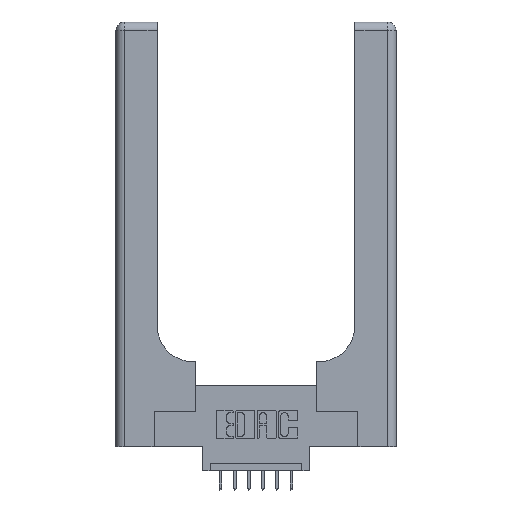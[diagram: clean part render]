
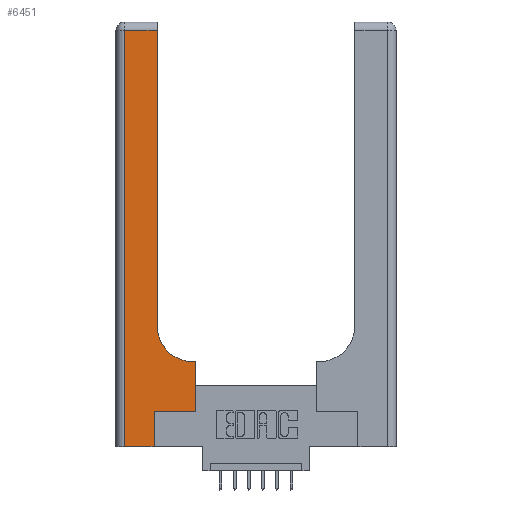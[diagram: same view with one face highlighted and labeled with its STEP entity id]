
A CAD part, top view. The second image highlights one B-rep face of the part: STEP entity #6451.
In plain terms, the highlighted planar face has unit normal (0, 0, 1).
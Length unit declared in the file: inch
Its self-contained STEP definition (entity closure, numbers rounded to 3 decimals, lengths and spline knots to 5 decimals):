
#187 = VECTOR ( 'NONE', #1304, 39.37008 ) ;
#385 = DIRECTION ( 'NONE',  ( -1., 0., 0. ) ) ;
#401 = LINE ( 'NONE', #9521, #187 ) ;
#418 = VECTOR ( 'NONE', #4972, 39.37008 ) ;
#908 = ORIENTED_EDGE ( 'NONE', *, *, #1554, .T. ) ;
#963 = VECTOR ( 'NONE', #2207, 39.37008 ) ;
#1245 = VECTOR ( 'NONE', #10351, 39.37008 ) ;
#1304 = DIRECTION ( 'NONE',  ( -1., 0., 0. ) ) ;
#1554 = EDGE_CURVE ( 'NONE', #9385, #5595, #4899, .T. ) ;
#1590 = VECTOR ( 'NONE', #8329, 39.37008 ) ;
#1761 = EDGE_LOOP ( 'NONE', ( #10314, #908, #6744, #7640, #12966, #4471, #8018, #3297, #11450 ) ) ;
#2207 = DIRECTION ( 'NONE',  ( 0., -1., 0. ) ) ;
#2430 = VECTOR ( 'NONE', #12287, 39.37008 ) ;
#2512 = CARTESIAN_POINT ( 'NONE',  ( 0.5415, 0.6, 0.37 ) ) ;
#2576 = CARTESIAN_POINT ( 'NONE',  ( 0.5585, 0.25, 0.37 ) ) ;
#2887 = CARTESIAN_POINT ( 'NONE',  ( 0.269, 0., 0.37 ) ) ;
#2919 = VERTEX_POINT ( 'NONE', #9083 ) ;
#3297 = ORIENTED_EDGE ( 'NONE', *, *, #8586, .T. ) ;
#3600 = CARTESIAN_POINT ( 'NONE',  ( 0.5585, 0.25, 0.37 ) ) ;
#4205 = VERTEX_POINT ( 'NONE', #2512 ) ;
#4418 = EDGE_CURVE ( 'NONE', #7313, #6484, #11014, .T. ) ;
#4419 = EDGE_CURVE ( 'NONE', #5595, #7313, #14674, .T. ) ;
#4471 = ORIENTED_EDGE ( 'NONE', *, *, #13167, .T. ) ;
#4771 = EDGE_CURVE ( 'NONE', #4205, #10143, #4777, .T. ) ;
#4777 = CIRCLE ( 'NONE', #7892, 0.25 ) ;
#4882 = CARTESIAN_POINT ( 'NONE',  ( 0.06, 0., 0.37 ) ) ;
#4899 = LINE ( 'NONE', #6180, #418 ) ;
#4972 = DIRECTION ( 'NONE',  ( -1., 0., 0. ) ) ;
#5291 = CARTESIAN_POINT ( 'NONE',  ( 0.06, 2.94, 0.37 ) ) ;
#5488 = LINE ( 'NONE', #8023, #9091 ) ;
#5595 = VERTEX_POINT ( 'NONE', #5291 ) ;
#5850 = CARTESIAN_POINT ( 'NONE',  ( 0.269, 0., 0.37 ) ) ;
#6180 = CARTESIAN_POINT ( 'NONE',  ( 0., 2.94, 0.37 ) ) ;
#6219 = CARTESIAN_POINT ( 'NONE',  ( 0.2915, 0.85, 0.37 ) ) ;
#6237 = LINE ( 'NONE', #2576, #1590 ) ;
#6451 = ADVANCED_FACE ( 'NONE', ( #8386 ), #8087, .F. ) ;
#6484 = VERTEX_POINT ( 'NONE', #5850 ) ;
#6689 = VECTOR ( 'NONE', #11310, 39.37008 ) ;
#6744 = ORIENTED_EDGE ( 'NONE', *, *, #4419, .T. ) ;
#7114 = CARTESIAN_POINT ( 'NONE',  ( 0., 3., 0.37 ) ) ;
#7195 = EDGE_CURVE ( 'NONE', #7717, #13067, #6237, .T. ) ;
#7313 = VERTEX_POINT ( 'NONE', #4882 ) ;
#7640 = ORIENTED_EDGE ( 'NONE', *, *, #4418, .T. ) ;
#7717 = VERTEX_POINT ( 'NONE', #3600 ) ;
#7733 = CARTESIAN_POINT ( 'NONE',  ( 0., 0., 0.37 ) ) ;
#7892 = AXIS2_PLACEMENT_3D ( 'NONE', #13038, #8564, #8709 ) ;
#8018 = ORIENTED_EDGE ( 'NONE', *, *, #7195, .T. ) ;
#8023 = CARTESIAN_POINT ( 'NONE',  ( 0.2915, 3., 0.37 ) ) ;
#8087 = PLANE ( 'NONE',  #10296 ) ;
#8329 = DIRECTION ( 'NONE',  ( 0., 1., 0. ) ) ;
#8386 = FACE_OUTER_BOUND ( 'NONE', #1761, .T. ) ;
#8564 = DIRECTION ( 'NONE',  ( 0., 0., -1. ) ) ;
#8586 = EDGE_CURVE ( 'NONE', #13067, #4205, #401, .T. ) ;
#8709 = DIRECTION ( 'NONE',  ( 1., 0., 0. ) ) ;
#9083 = CARTESIAN_POINT ( 'NONE',  ( 0.269, 0.25, 0.37 ) ) ;
#9091 = VECTOR ( 'NONE', #12567, 39.37008 ) ;
#9385 = VERTEX_POINT ( 'NONE', #14555 ) ;
#9521 = CARTESIAN_POINT ( 'NONE',  ( 0.2915, 0.6, 0.37 ) ) ;
#9967 = LINE ( 'NONE', #2887, #2430 ) ;
#10042 = CARTESIAN_POINT ( 'NONE',  ( 0.06, 3., 0.37 ) ) ;
#10065 = CARTESIAN_POINT ( 'NONE',  ( 0.269, 0.25, 0.37 ) ) ;
#10143 = VERTEX_POINT ( 'NONE', #6219 ) ;
#10296 = AXIS2_PLACEMENT_3D ( 'NONE', #7114, #10544, #385 ) ;
#10314 = ORIENTED_EDGE ( 'NONE', *, *, #12494, .T. ) ;
#10351 = DIRECTION ( 'NONE',  ( 1., 0., 0. ) ) ;
#10544 = DIRECTION ( 'NONE',  ( 0., 0., -1. ) ) ;
#11014 = LINE ( 'NONE', #7733, #6689 ) ;
#11310 = DIRECTION ( 'NONE',  ( 1., 0., 0. ) ) ;
#11328 = LINE ( 'NONE', #10065, #1245 ) ;
#11450 = ORIENTED_EDGE ( 'NONE', *, *, #4771, .T. ) ;
#12080 = CARTESIAN_POINT ( 'NONE',  ( 0.5585, 0.6, 0.37 ) ) ;
#12287 = DIRECTION ( 'NONE',  ( 0., 1., 0. ) ) ;
#12494 = EDGE_CURVE ( 'NONE', #10143, #9385, #5488, .T. ) ;
#12567 = DIRECTION ( 'NONE',  ( 0., 1., 0. ) ) ;
#12966 = ORIENTED_EDGE ( 'NONE', *, *, #14648, .T. ) ;
#13038 = CARTESIAN_POINT ( 'NONE',  ( 0.5415, 0.85, 0.37 ) ) ;
#13067 = VERTEX_POINT ( 'NONE', #12080 ) ;
#13167 = EDGE_CURVE ( 'NONE', #2919, #7717, #11328, .T. ) ;
#14555 = CARTESIAN_POINT ( 'NONE',  ( 0.2915, 2.94, 0.37 ) ) ;
#14648 = EDGE_CURVE ( 'NONE', #6484, #2919, #9967, .T. ) ;
#14674 = LINE ( 'NONE', #10042, #963 ) ;
